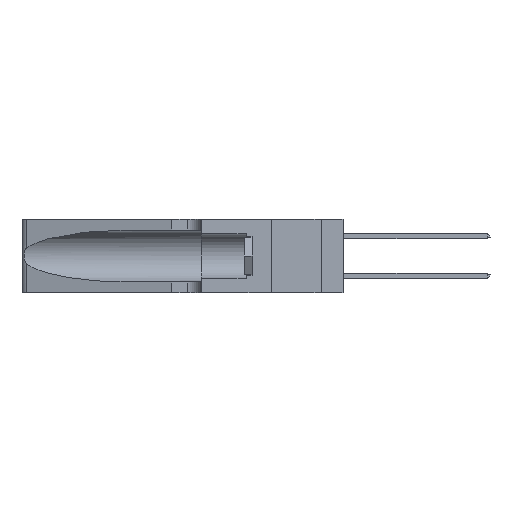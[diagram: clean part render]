
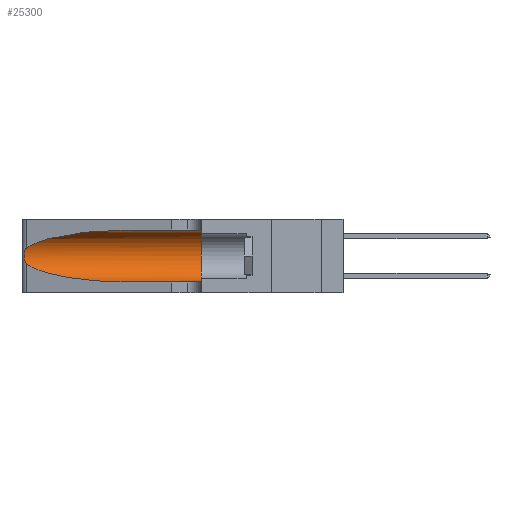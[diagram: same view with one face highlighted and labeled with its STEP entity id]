
A CAD part, left-side view. The second image highlights one B-rep face of the part: STEP entity #25300.
In plain terms, the highlighted cylindrical face has radius 3.308 mm (diameter 6.617 mm), a partial arc.
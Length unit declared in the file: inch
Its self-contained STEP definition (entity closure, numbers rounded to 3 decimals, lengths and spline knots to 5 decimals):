
#485 = VECTOR ( 'NONE', #27066, 39.37008 ) ;
#641 = ORIENTED_EDGE ( 'NONE', *, *, #26551, .T. ) ;
#943 = EDGE_CURVE ( 'NONE', #24318, #2940, #17446, .T. ) ;
#1327 =( BOUNDED_CURVE ( )  B_SPLINE_CURVE ( 3, ( #9169, #26319, #32027, #14949 ),
 .UNSPECIFIED., .F., .F. ) 
 B_SPLINE_CURVE_WITH_KNOTS ( ( 4, 4 ),
 ( 1.5708, 2.84003 ),
 .UNSPECIFIED. ) 
 CURVE ( )  GEOMETRIC_REPRESENTATION_ITEM ( )  RATIONAL_B_SPLINE_CURVE ( ( 1., 0.87, 0.87, 1. ) ) 
 REPRESENTATION_ITEM ( '' )  );
#1590 = CARTESIAN_POINT ( 'NONE',  ( 0.25555, 1.22993, 0.14849 ) ) ;
#1789 = CIRCLE ( 'NONE', #12778, 0.13025 ) ;
#1849 = VERTEX_POINT ( 'NONE', #4672 ) ;
#2283 = EDGE_CURVE ( 'NONE', #9444, #14940, #17454, .T. ) ;
#2940 = VERTEX_POINT ( 'NONE', #7191 ) ;
#3334 = CARTESIAN_POINT ( 'NONE',  ( 0.2373, 1.15595, 0.08982 ) ) ;
#4141 = CARTESIAN_POINT ( 'NONE',  ( 0.1305, 1.61858, 0.05475 ) ) ;
#4607 = DIRECTION ( 'NONE',  ( 0., -1., 0. ) ) ;
#4672 = CARTESIAN_POINT ( 'NONE',  ( 0.1305, 0.35, 0.05475 ) ) ;
#5121 = VERTEX_POINT ( 'NONE', #12836 ) ;
#6208 = CARTESIAN_POINT ( 'NONE',  ( 0.18966, 0.96281, 0.05475 ) ) ;
#6682 = AXIS2_PLACEMENT_3D ( 'NONE', #18386, #26987, #6939 ) ;
#6828 = CYLINDRICAL_SURFACE ( 'NONE', #6682, 0.13025 ) ;
#6939 = DIRECTION ( 'NONE',  ( 0., 0., -1. ) ) ;
#7191 = CARTESIAN_POINT ( 'NONE',  ( 0.1305, 0.72297, 0.05475 ) ) ;
#7238 = CARTESIAN_POINT ( 'NONE',  ( 0.25787, 1.23484, 0.2124 ) ) ;
#9169 = CARTESIAN_POINT ( 'NONE',  ( 0.1305, 0.72297, 0.31525 ) ) ;
#9444 = VERTEX_POINT ( 'NONE', #31774 ) ;
#9704 = ORIENTED_EDGE ( 'NONE', *, *, #2283, .F. ) ;
#10153 = CARTESIAN_POINT ( 'NONE',  ( 0.26018, 1.23835, 0.19895 ) ) ;
#12379 = ORIENTED_EDGE ( 'NONE', *, *, #27032, .F. ) ;
#12778 = AXIS2_PLACEMENT_3D ( 'NONE', #17054, #36961, #19953 ) ;
#12836 = CARTESIAN_POINT ( 'NONE',  ( 0.25487, 1.22718, 0.22369 ) ) ;
#12918 = CARTESIAN_POINT ( 'NONE',  ( 0.25555, 1.22994, 0.2215 ) ) ;
#13048 = CARTESIAN_POINT ( 'NONE',  ( 0.26075, 1.23896, 0.178 ) ) ;
#14894 = LINE ( 'NONE', #4141, #485 ) ;
#14940 = VERTEX_POINT ( 'NONE', #17878 ) ;
#14949 = CARTESIAN_POINT ( 'NONE',  ( 0.25487, 1.22718, 0.22369 ) ) ;
#15899 = CARTESIAN_POINT ( 'NONE',  ( 0.25856, 1.23593, 0.16098 ) ) ;
#16373 = EDGE_CURVE ( 'NONE', #5121, #24318, #27966, .T. ) ;
#17054 = CARTESIAN_POINT ( 'NONE',  ( 0.1305, 0.35, 0.185 ) ) ;
#17171 = ORIENTED_EDGE ( 'NONE', *, *, #25995, .T. ) ;
#17446 =( BOUNDED_CURVE ( )  B_SPLINE_CURVE ( 3, ( #23389, #3334, #6208, #26251 ),
 .UNSPECIFIED., .F., .F. ) 
 B_SPLINE_CURVE_WITH_KNOTS ( ( 4, 4 ),
 ( 3.44316, 4.71239 ),
 .UNSPECIFIED. ) 
 CURVE ( )  GEOMETRIC_REPRESENTATION_ITEM ( )  RATIONAL_B_SPLINE_CURVE ( ( 1., 0.87, 0.87, 1. ) ) 
 REPRESENTATION_ITEM ( '' )  );
#17454 = LINE ( 'NONE', #21786, #32634 ) ;
#17878 = CARTESIAN_POINT ( 'NONE',  ( 0.1305, 0.35, 0.31525 ) ) ;
#18386 = CARTESIAN_POINT ( 'NONE',  ( 0.1305, 1.61858, 0.185 ) ) ;
#18676 = CARTESIAN_POINT ( 'NONE',  ( 0.25487, 1.22718, 0.22369 ) ) ;
#18810 = CARTESIAN_POINT ( 'NONE',  ( 0.25639, 1.23186, 0.15144 ) ) ;
#19953 = DIRECTION ( 'NONE',  ( 0., 0., 1. ) ) ;
#21670 = CARTESIAN_POINT ( 'NONE',  ( 0.25487, 1.22718, 0.14631 ) ) ;
#21786 = CARTESIAN_POINT ( 'NONE',  ( 0.1305, 1.61858, 0.31525 ) ) ;
#22110 = FACE_OUTER_BOUND ( 'NONE', #29289, .T. ) ;
#23389 = CARTESIAN_POINT ( 'NONE',  ( 0.25487, 1.22718, 0.14631 ) ) ;
#24318 = VERTEX_POINT ( 'NONE', #34399 ) ;
#24401 = CARTESIAN_POINT ( 'NONE',  ( 0.25639, 1.23184, 0.21858 ) ) ;
#25300 = ADVANCED_FACE ( 'NONE', ( #22110 ), #6828, .F. ) ;
#25598 = ORIENTED_EDGE ( 'NONE', *, *, #16373, .T. ) ;
#25995 = EDGE_CURVE ( 'NONE', #2940, #1849, #14894, .T. ) ;
#26251 = CARTESIAN_POINT ( 'NONE',  ( 0.1305, 0.72297, 0.05475 ) ) ;
#26319 = CARTESIAN_POINT ( 'NONE',  ( 0.18966, 0.96281, 0.31525 ) ) ;
#26551 = EDGE_CURVE ( 'NONE', #9444, #5121, #1327, .T. ) ;
#26987 = DIRECTION ( 'NONE',  ( 0., -1., 0. ) ) ;
#27032 = EDGE_CURVE ( 'NONE', #14940, #1849, #1789, .T. ) ;
#27066 = DIRECTION ( 'NONE',  ( 0., -1., 0. ) ) ;
#27274 = CARTESIAN_POINT ( 'NONE',  ( 0.25854, 1.2359, 0.20912 ) ) ;
#27966 = B_SPLINE_CURVE_WITH_KNOTS ( 'NONE', 3,
 ( #18676, #12918, #24401, #7238, #27274, #10153, #30151, #13048, #33014, #15899, #35834, #18810, #1590, #21670 ),
 .UNSPECIFIED., .F., .F.,
 ( 4, 2, 2, 2, 2, 2, 4 ),
 ( 0., 0.00027, 0.00053, 0.00107, 0.0016, 0.00187, 0.00214 ),
 .UNSPECIFIED. ) ;
#29289 = EDGE_LOOP ( 'NONE', ( #641, #25598, #35015, #17171, #12379, #9704 ) ) ;
#30151 = CARTESIAN_POINT ( 'NONE',  ( 0.26075, 1.23896, 0.19203 ) ) ;
#31774 = CARTESIAN_POINT ( 'NONE',  ( 0.1305, 0.72297, 0.31525 ) ) ;
#32027 = CARTESIAN_POINT ( 'NONE',  ( 0.2373, 1.15595, 0.28018 ) ) ;
#32634 = VECTOR ( 'NONE', #4607, 39.37008 ) ;
#33014 = CARTESIAN_POINT ( 'NONE',  ( 0.26017, 1.23833, 0.17102 ) ) ;
#34399 = CARTESIAN_POINT ( 'NONE',  ( 0.25487, 1.22718, 0.14631 ) ) ;
#35015 = ORIENTED_EDGE ( 'NONE', *, *, #943, .T. ) ;
#35834 = CARTESIAN_POINT ( 'NONE',  ( 0.25789, 1.23486, 0.15765 ) ) ;
#36961 = DIRECTION ( 'NONE',  ( 0., 1., 0. ) ) ;
